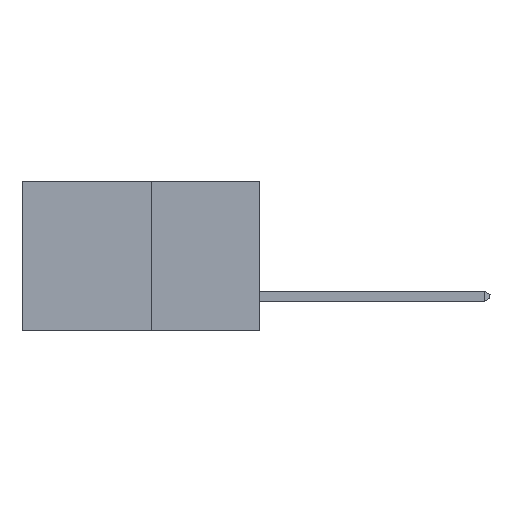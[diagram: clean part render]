
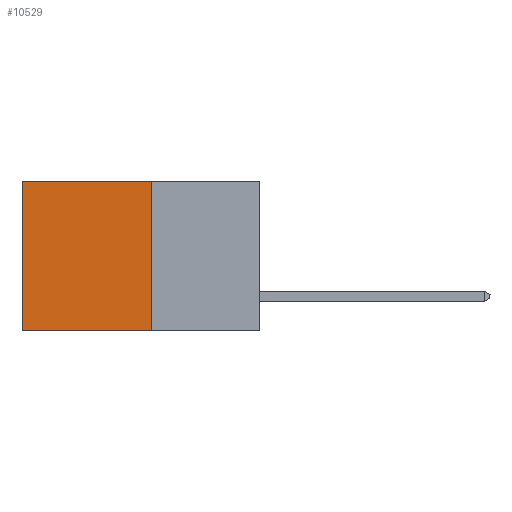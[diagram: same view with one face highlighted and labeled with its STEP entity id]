
A CAD part, left-side view. The second image highlights one B-rep face of the part: STEP entity #10529.
In plain terms, the highlighted planar face has unit normal (-1, 0, 0).
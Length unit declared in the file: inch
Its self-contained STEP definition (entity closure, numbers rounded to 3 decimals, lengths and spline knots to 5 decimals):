
#479 = VERTEX_POINT ( 'NONE', #17755 ) ;
#1518 = VECTOR ( 'NONE', #5338, 39.37008 ) ;
#2702 = VECTOR ( 'NONE', #11127, 39.37008 ) ;
#2859 = DIRECTION ( 'NONE',  ( 1., 0., 0. ) ) ;
#3372 = ORIENTED_EDGE ( 'NONE', *, *, #14715, .F. ) ;
#4491 = CARTESIAN_POINT ( 'NONE',  ( 0.277, 0.59, -0.37 ) ) ;
#5338 = DIRECTION ( 'NONE',  ( 0., 1., 0. ) ) ;
#5375 = ORIENTED_EDGE ( 'NONE', *, *, #25867, .T. ) ;
#5872 = CARTESIAN_POINT ( 'NONE',  ( 0.277, 0.59, 0. ) ) ;
#6031 = LINE ( 'NONE', #11480, #22015 ) ;
#8419 = LINE ( 'NONE', #4491, #2702 ) ;
#9626 = ORIENTED_EDGE ( 'NONE', *, *, #25126, .T. ) ;
#9969 = VERTEX_POINT ( 'NONE', #5872 ) ;
#10529 = ADVANCED_FACE ( 'NONE', ( #21103 ), #10554, .F. ) ;
#10554 = PLANE ( 'NONE',  #22808 ) ;
#11127 = DIRECTION ( 'NONE',  ( 0., 0., -1. ) ) ;
#11276 = EDGE_CURVE ( 'NONE', #24256, #13199, #22785, .T. ) ;
#11480 = CARTESIAN_POINT ( 'NONE',  ( 0.277, 0.27, 0. ) ) ;
#11685 = CARTESIAN_POINT ( 'NONE',  ( 0.277, 0.27, -0.37 ) ) ;
#12993 = EDGE_LOOP ( 'NONE', ( #9626, #3372, #25621, #5375 ) ) ;
#13199 = VERTEX_POINT ( 'NONE', #20487 ) ;
#13656 = DIRECTION ( 'NONE',  ( 0., 1., 0. ) ) ;
#14715 = EDGE_CURVE ( 'NONE', #13199, #479, #23235, .T. ) ;
#16140 = CARTESIAN_POINT ( 'NONE',  ( 0.277, 0.27, -0.37 ) ) ;
#16968 = VECTOR ( 'NONE', #20389, 39.37008 ) ;
#17755 = CARTESIAN_POINT ( 'NONE',  ( 0.277, 0.59, -0.37 ) ) ;
#18284 = DIRECTION ( 'NONE',  ( 0., 0., -1. ) ) ;
#20389 = DIRECTION ( 'NONE',  ( 0., 0., -1. ) ) ;
#20487 = CARTESIAN_POINT ( 'NONE',  ( 0.277, 0.27, -0.37 ) ) ;
#20760 = CARTESIAN_POINT ( 'NONE',  ( 0.277, 0.27, -0.37 ) ) ;
#21103 = FACE_OUTER_BOUND ( 'NONE', #12993, .T. ) ;
#22015 = VECTOR ( 'NONE', #13656, 39.37008 ) ;
#22785 = LINE ( 'NONE', #20760, #16968 ) ;
#22808 = AXIS2_PLACEMENT_3D ( 'NONE', #11685, #2859, #18284 ) ;
#23235 = LINE ( 'NONE', #16140, #1518 ) ;
#24256 = VERTEX_POINT ( 'NONE', #27773 ) ;
#25126 = EDGE_CURVE ( 'NONE', #9969, #479, #8419, .T. ) ;
#25621 = ORIENTED_EDGE ( 'NONE', *, *, #11276, .F. ) ;
#25867 = EDGE_CURVE ( 'NONE', #24256, #9969, #6031, .T. ) ;
#27773 = CARTESIAN_POINT ( 'NONE',  ( 0.277, 0.27, 0. ) ) ;
